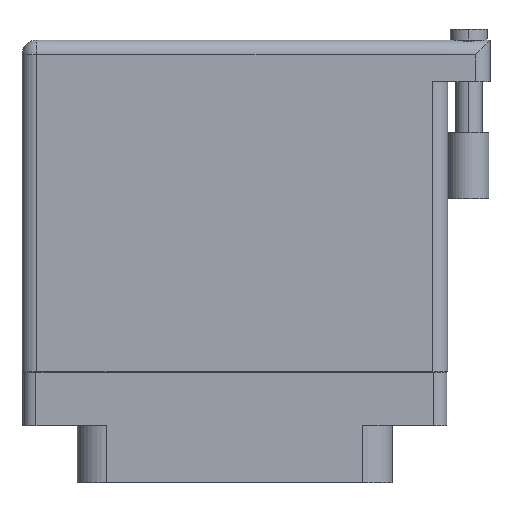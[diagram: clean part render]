
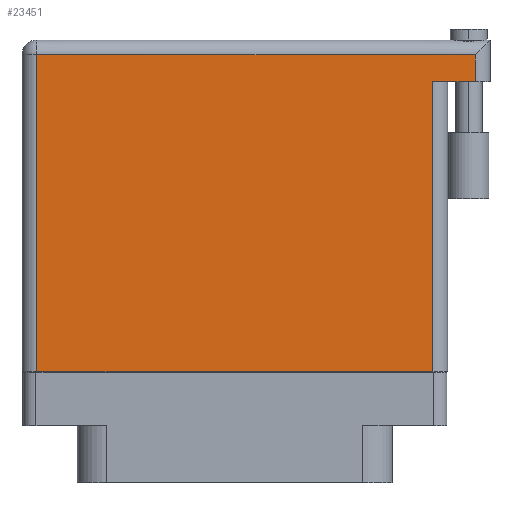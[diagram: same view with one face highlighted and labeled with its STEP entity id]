
A CAD part, front view. The second image highlights one B-rep face of the part: STEP entity #23451.
In plain terms, the highlighted face is planar.
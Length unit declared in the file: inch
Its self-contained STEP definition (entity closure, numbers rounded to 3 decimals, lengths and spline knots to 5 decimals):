
#276 = VECTOR ( 'NONE', #15115, 39.37008 ) ;
#355 = ORIENTED_EDGE ( 'NONE', *, *, #22090, .T. ) ;
#1184 = CARTESIAN_POINT ( 'NONE',  ( -1.004, 1.466, 0.4495 ) ) ;
#1299 = DIRECTION ( 'NONE',  ( -1., 0., 0. ) ) ;
#1965 = VECTOR ( 'NONE', #15116, 39.37008 ) ;
#3476 = VERTEX_POINT ( 'NONE', #3803 ) ;
#3803 = CARTESIAN_POINT ( 'NONE',  ( 0.934, -0.1, 0.4495 ) ) ;
#3970 = VERTEX_POINT ( 'NONE', #13204 ) ;
#5173 = CARTESIAN_POINT ( 'NONE',  ( 1.134, 1.466, 0.4495 ) ) ;
#8225 = LINE ( 'NONE', #10587, #34523 ) ;
#8981 = EDGE_CURVE ( 'NONE', #30494, #24103, #20157, .T. ) ;
#9712 = CARTESIAN_POINT ( 'NONE',  ( -1.004, 1.396, 0.4495 ) ) ;
#10288 = DIRECTION ( 'NONE',  ( -1., 0., 0. ) ) ;
#10587 = CARTESIAN_POINT ( 'NONE',  ( -1.004, -0.1, 0.4495 ) ) ;
#10716 = DIRECTION ( 'NONE',  ( 0., 1., 0. ) ) ;
#11937 = FACE_OUTER_BOUND ( 'NONE', #26075, .T. ) ;
#13204 = CARTESIAN_POINT ( 'NONE',  ( 1.134, 1.396, 0.4495 ) ) ;
#15115 = DIRECTION ( 'NONE',  ( -1., 0., 0. ) ) ;
#15116 = DIRECTION ( 'NONE',  ( 0., -1., 0. ) ) ;
#15692 = DIRECTION ( 'NONE',  ( 0., 1., 0. ) ) ;
#15752 = CARTESIAN_POINT ( 'NONE',  ( 1.134, 1.269, 0.4495 ) ) ;
#16100 = ORIENTED_EDGE ( 'NONE', *, *, #20738, .T. ) ;
#16734 = CARTESIAN_POINT ( 'NONE',  ( -0.934, 1.396, 0.4495 ) ) ;
#17947 = EDGE_CURVE ( 'NONE', #33716, #3476, #8225, .T. ) ;
#20157 = LINE ( 'NONE', #26989, #26589 ) ;
#20610 = EDGE_CURVE ( 'NONE', #30494, #3970, #25667, .T. ) ;
#20713 = PLANE ( 'NONE',  #21867 ) ;
#20738 = EDGE_CURVE ( 'NONE', #30115, #33716, #33040, .T. ) ;
#21867 = AXIS2_PLACEMENT_3D ( 'NONE', #1184, #25762, #1299 ) ;
#22090 = EDGE_CURVE ( 'NONE', #3476, #24103, #33976, .T. ) ;
#23303 = ORIENTED_EDGE ( 'NONE', *, *, #20610, .T. ) ;
#23451 = ADVANCED_FACE ( 'NONE', ( #11937 ), #20713, .F. ) ;
#23673 = ORIENTED_EDGE ( 'NONE', *, *, #23851, .T. ) ;
#23851 = EDGE_CURVE ( 'NONE', #3970, #30115, #34330, .T. ) ;
#24103 = VERTEX_POINT ( 'NONE', #33075 ) ;
#25667 = LINE ( 'NONE', #5173, #29131 ) ;
#25762 = DIRECTION ( 'NONE',  ( 0., 0., -1. ) ) ;
#26075 = EDGE_LOOP ( 'NONE', ( #28102, #355, #34918, #23303, #23673, #16100 ) ) ;
#26388 = CARTESIAN_POINT ( 'NONE',  ( 0.934, 1.269, 0.4495 ) ) ;
#26589 = VECTOR ( 'NONE', #10288, 39.37008 ) ;
#26989 = CARTESIAN_POINT ( 'NONE',  ( 1.204, 1.269, 0.4495 ) ) ;
#27503 = VECTOR ( 'NONE', #15692, 39.37008 ) ;
#28102 = ORIENTED_EDGE ( 'NONE', *, *, #17947, .T. ) ;
#29131 = VECTOR ( 'NONE', #10716, 39.37008 ) ;
#29482 = DIRECTION ( 'NONE',  ( 1., 0., 0. ) ) ;
#29570 = CARTESIAN_POINT ( 'NONE',  ( -0.934, -0.1, 0.4495 ) ) ;
#30115 = VERTEX_POINT ( 'NONE', #16734 ) ;
#30494 = VERTEX_POINT ( 'NONE', #15752 ) ;
#31636 = CARTESIAN_POINT ( 'NONE',  ( -0.934, -0.1, 0.4495 ) ) ;
#33040 = LINE ( 'NONE', #31636, #1965 ) ;
#33075 = CARTESIAN_POINT ( 'NONE',  ( 0.934, 1.269, 0.4495 ) ) ;
#33716 = VERTEX_POINT ( 'NONE', #29570 ) ;
#33976 = LINE ( 'NONE', #26388, #27503 ) ;
#34330 = LINE ( 'NONE', #9712, #276 ) ;
#34523 = VECTOR ( 'NONE', #29482, 39.37008 ) ;
#34918 = ORIENTED_EDGE ( 'NONE', *, *, #8981, .F. ) ;
